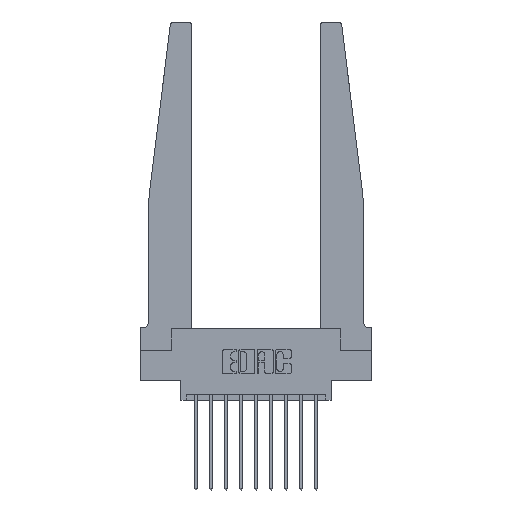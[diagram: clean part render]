
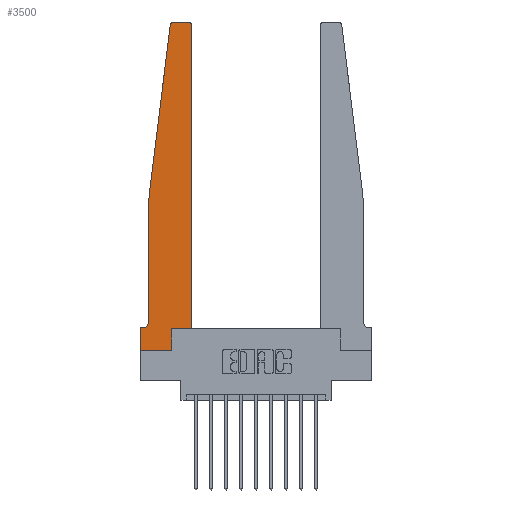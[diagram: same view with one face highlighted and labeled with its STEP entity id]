
A CAD part, top view. The second image highlights one B-rep face of the part: STEP entity #3500.
In plain terms, the highlighted planar face has unit normal (0, 0, 1).
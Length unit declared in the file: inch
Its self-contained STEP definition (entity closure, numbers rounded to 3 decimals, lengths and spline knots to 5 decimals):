
#254 = ORIENTED_EDGE ( 'NONE', *, *, #13064, .T. ) ;
#523 = CARTESIAN_POINT ( 'NONE',  ( 0.27653, 2.75, 0.37 ) ) ;
#679 = EDGE_CURVE ( 'NONE', #11729, #8891, #12743, .T. ) ;
#790 = EDGE_CURVE ( 'NONE', #3834, #3928, #7340, .T. ) ;
#822 = VECTOR ( 'NONE', #15425, 39.37008 ) ;
#831 = CARTESIAN_POINT ( 'NONE',  ( 0.395, 2.72, 0.37 ) ) ;
#1260 = CARTESIAN_POINT ( 'NONE',  ( 0., 0.1875, 0.37 ) ) ;
#1445 = DIRECTION ( 'NONE',  ( 0., -1., 0. ) ) ;
#1456 = CARTESIAN_POINT ( 'NONE',  ( 0.2605, 0., 0.37 ) ) ;
#1780 = DIRECTION ( 'NONE',  ( 0., 0., 1. ) ) ;
#1896 = DIRECTION ( 'NONE',  ( 1., 0., 0. ) ) ;
#1912 = VECTOR ( 'NONE', #10439, 39.37008 ) ;
#2022 = CARTESIAN_POINT ( 'NONE',  ( 0.015, 0.2375, 0.37 ) ) ;
#2028 = DIRECTION ( 'NONE',  ( 1., 0., 0. ) ) ;
#2074 = VECTOR ( 'NONE', #4463, 39.37008 ) ;
#2379 = VERTEX_POINT ( 'NONE', #7701 ) ;
#2461 = CARTESIAN_POINT ( 'NONE',  ( 0.395, 2.75, 0.37 ) ) ;
#2620 = ORIENTED_EDGE ( 'NONE', *, *, #679, .T. ) ;
#2815 = VERTEX_POINT ( 'NONE', #10057 ) ;
#2946 = DIRECTION ( 'NONE',  ( 0., 1., 0. ) ) ;
#3007 = VECTOR ( 'NONE', #1445, 39.37008 ) ;
#3210 = ORIENTED_EDGE ( 'NONE', *, *, #790, .T. ) ;
#3487 = EDGE_CURVE ( 'NONE', #11869, #7780, #9162, .T. ) ;
#3500 = ADVANCED_FACE ( 'NONE', ( #15426 ), #15271, .T. ) ;
#3687 = EDGE_CURVE ( 'NONE', #8891, #8898, #11050, .T. ) ;
#3834 = VERTEX_POINT ( 'NONE', #7149 ) ;
#3928 = VERTEX_POINT ( 'NONE', #1260 ) ;
#4103 = ORIENTED_EDGE ( 'NONE', *, *, #13294, .T. ) ;
#4278 = LINE ( 'NONE', #5298, #8155 ) ;
#4384 = VECTOR ( 'NONE', #12161, 39.37008 ) ;
#4463 = DIRECTION ( 'NONE',  ( 1., 0., 0. ) ) ;
#4481 = DIRECTION ( 'NONE',  ( 0., 0., -1. ) ) ;
#4662 = LINE ( 'NONE', #11948, #7622 ) ;
#5096 = DIRECTION ( 'NONE',  ( 0., 1., 0. ) ) ;
#5244 = ORIENTED_EDGE ( 'NONE', *, *, #8441, .T. ) ;
#5298 = CARTESIAN_POINT ( 'NONE',  ( 0.2605, 0.18, 0.37 ) ) ;
#5885 = CARTESIAN_POINT ( 'NONE',  ( 0., 0., 0.37 ) ) ;
#5980 = CARTESIAN_POINT ( 'NONE',  ( 0.2605, 0.18, 0.37 ) ) ;
#6100 = VERTEX_POINT ( 'NONE', #1456 ) ;
#6807 = CARTESIAN_POINT ( 'NONE',  ( 0.065, 0.1875, 0.37 ) ) ;
#6855 = DIRECTION ( 'NONE',  ( -1., 0., 0. ) ) ;
#6856 = DIRECTION ( 'NONE',  ( 0., 0., 1. ) ) ;
#6917 = VECTOR ( 'NONE', #1896, 39.37008 ) ;
#7149 = CARTESIAN_POINT ( 'NONE',  ( 0.015, 0.1875, 0.37 ) ) ;
#7340 = LINE ( 'NONE', #6807, #4384 ) ;
#7622 = VECTOR ( 'NONE', #15354, 39.37008 ) ;
#7636 = CIRCLE ( 'NONE', #11167, 0.03 ) ;
#7670 = CIRCLE ( 'NONE', #13742, 0.05 ) ;
#7701 = CARTESIAN_POINT ( 'NONE',  ( 0.065, 0.2375, 0.37 ) ) ;
#7780 = VERTEX_POINT ( 'NONE', #523 ) ;
#8155 = VECTOR ( 'NONE', #2946, 39.37008 ) ;
#8441 = EDGE_CURVE ( 'NONE', #15411, #2379, #8596, .T. ) ;
#8596 = LINE ( 'NONE', #13427, #3007 ) ;
#8803 = CARTESIAN_POINT ( 'NONE',  ( 0.425, 2.72, 0.37 ) ) ;
#8891 = VERTEX_POINT ( 'NONE', #14837 ) ;
#8898 = VERTEX_POINT ( 'NONE', #8803 ) ;
#9162 = LINE ( 'NONE', #13918, #1912 ) ;
#9685 = EDGE_CURVE ( 'NONE', #7780, #2815, #10880, .T. ) ;
#9919 = VERTEX_POINT ( 'NONE', #5885 ) ;
#9944 = DIRECTION ( 'NONE',  ( 0., 0., 1. ) ) ;
#10057 = CARTESIAN_POINT ( 'NONE',  ( 0.24675, 2.72367, 0.37 ) ) ;
#10096 = CARTESIAN_POINT ( 'NONE',  ( 0.425, 0.18, 0.37 ) ) ;
#10439 = DIRECTION ( 'NONE',  ( -1., 0., 0. ) ) ;
#10574 = LINE ( 'NONE', #14057, #2074 ) ;
#10679 = LINE ( 'NONE', #13053, #822 ) ;
#10880 = CIRCLE ( 'NONE', #13419, 0.03 ) ;
#10970 = CARTESIAN_POINT ( 'NONE',  ( 0.27653, 2.72, 0.37 ) ) ;
#11009 = VECTOR ( 'NONE', #5096, 39.37008 ) ;
#11050 = LINE ( 'NONE', #10096, #11009 ) ;
#11118 = EDGE_CURVE ( 'NONE', #3928, #9919, #4662, .T. ) ;
#11167 = AXIS2_PLACEMENT_3D ( 'NONE', #831, #6856, #13049 ) ;
#11729 = VERTEX_POINT ( 'NONE', #5980 ) ;
#11869 = VERTEX_POINT ( 'NONE', #2461 ) ;
#11948 = CARTESIAN_POINT ( 'NONE',  ( 0., 0., 0.37 ) ) ;
#12161 = DIRECTION ( 'NONE',  ( -1., 0., 0. ) ) ;
#12743 = LINE ( 'NONE', #14980, #6917 ) ;
#12794 = EDGE_CURVE ( 'NONE', #8898, #11869, #7636, .T. ) ;
#12875 = CARTESIAN_POINT ( 'NONE',  ( 0., 0.1875, 0.37 ) ) ;
#13049 = DIRECTION ( 'NONE',  ( 1., 0., 0. ) ) ;
#13053 = CARTESIAN_POINT ( 'NONE',  ( 0.065, 1.25, 0.37 ) ) ;
#13055 = ORIENTED_EDGE ( 'NONE', *, *, #13878, .T. ) ;
#13064 = EDGE_CURVE ( 'NONE', #9919, #6100, #10574, .T. ) ;
#13245 = ORIENTED_EDGE ( 'NONE', *, *, #3487, .T. ) ;
#13294 = EDGE_CURVE ( 'NONE', #6100, #11729, #4278, .T. ) ;
#13316 = ORIENTED_EDGE ( 'NONE', *, *, #14566, .T. ) ;
#13419 = AXIS2_PLACEMENT_3D ( 'NONE', #10970, #9944, #14781 ) ;
#13427 = CARTESIAN_POINT ( 'NONE',  ( 0.065, 1.25, 0.37 ) ) ;
#13742 = AXIS2_PLACEMENT_3D ( 'NONE', #2022, #4481, #6855 ) ;
#13758 = CARTESIAN_POINT ( 'NONE',  ( 0.065, 1.25, 0.37 ) ) ;
#13878 = EDGE_CURVE ( 'NONE', #2815, #15411, #10679, .T. ) ;
#13918 = CARTESIAN_POINT ( 'NONE',  ( 0.25, 2.75, 0.37 ) ) ;
#14057 = CARTESIAN_POINT ( 'NONE',  ( 0., 0., 0.37 ) ) ;
#14330 = AXIS2_PLACEMENT_3D ( 'NONE', #12875, #1780, #2028 ) ;
#14431 = ORIENTED_EDGE ( 'NONE', *, *, #9685, .T. ) ;
#14566 = EDGE_CURVE ( 'NONE', #2379, #3834, #7670, .T. ) ;
#14727 = ORIENTED_EDGE ( 'NONE', *, *, #11118, .T. ) ;
#14781 = DIRECTION ( 'NONE',  ( 1., 0., 0. ) ) ;
#14837 = CARTESIAN_POINT ( 'NONE',  ( 0.425, 0.18, 0.37 ) ) ;
#14980 = CARTESIAN_POINT ( 'NONE',  ( 0.425, 0.18, 0.37 ) ) ;
#15069 = EDGE_LOOP ( 'NONE', ( #13245, #14431, #13055, #5244, #13316, #3210, #14727, #254, #4103, #2620, #15364, #15562 ) ) ;
#15271 = PLANE ( 'NONE',  #14330 ) ;
#15354 = DIRECTION ( 'NONE',  ( 0., -1., 0. ) ) ;
#15364 = ORIENTED_EDGE ( 'NONE', *, *, #3687, .T. ) ;
#15411 = VERTEX_POINT ( 'NONE', #13758 ) ;
#15425 = DIRECTION ( 'NONE',  ( -0.122, -0.992, 0. ) ) ;
#15426 = FACE_OUTER_BOUND ( 'NONE', #15069, .T. ) ;
#15562 = ORIENTED_EDGE ( 'NONE', *, *, #12794, .T. ) ;
